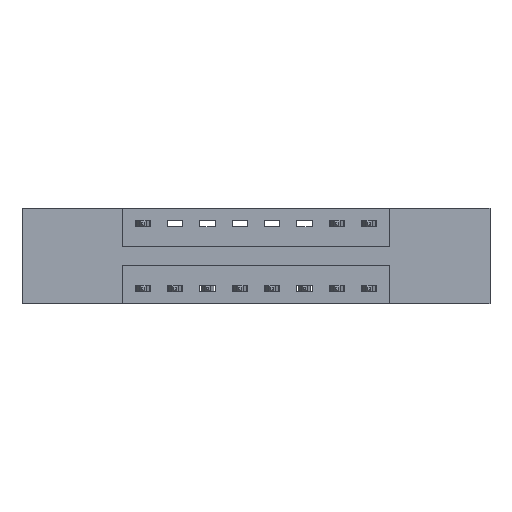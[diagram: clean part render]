
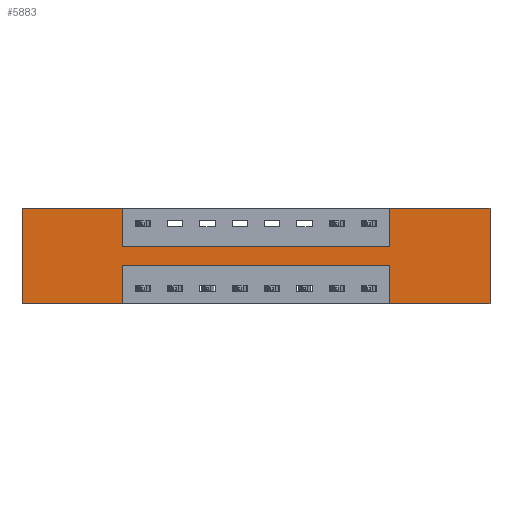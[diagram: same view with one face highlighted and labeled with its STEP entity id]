
A CAD part, front view. The second image highlights one B-rep face of the part: STEP entity #5883.
In plain terms, the highlighted planar face has unit normal (0, -1, 0).
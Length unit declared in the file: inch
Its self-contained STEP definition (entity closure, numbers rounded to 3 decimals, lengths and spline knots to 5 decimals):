
#243 = ORIENTED_EDGE ( 'NONE', *, *, #7865, .F. ) ;
#337 = EDGE_CURVE ( 'NONE', #3674, #3912, #1837, .T. ) ;
#371 = VECTOR ( 'NONE', #8137, 39.37008 ) ;
#409 = VECTOR ( 'NONE', #5251, 39.37008 ) ;
#475 = LINE ( 'NONE', #8628, #8209 ) ;
#596 = VECTOR ( 'NONE', #3770, 39.37008 ) ;
#738 = DIRECTION ( 'NONE',  ( 1., 0., 0. ) ) ;
#795 = CARTESIAN_POINT ( 'NONE',  ( 0.3875, 0., 0. ) ) ;
#803 = CARTESIAN_POINT ( 'NONE',  ( 0., 0., 0. ) ) ;
#1047 = ORIENTED_EDGE ( 'NONE', *, *, #8510, .F. ) ;
#1082 = CARTESIAN_POINT ( 'NONE',  ( 0.3875, 0., -0.37 ) ) ;
#1118 = DIRECTION ( 'NONE',  ( 1., 0., 0. ) ) ;
#1181 = FACE_OUTER_BOUND ( 'NONE', #6843, .T. ) ;
#1190 = ORIENTED_EDGE ( 'NONE', *, *, #1732, .F. ) ;
#1192 = LINE ( 'NONE', #1082, #5356 ) ;
#1216 = ORIENTED_EDGE ( 'NONE', *, *, #2762, .F. ) ;
#1346 = CARTESIAN_POINT ( 'NONE',  ( 0.3875, 0., 0. ) ) ;
#1477 = CARTESIAN_POINT ( 'NONE',  ( 0.3875, 0., -0.22 ) ) ;
#1499 = CARTESIAN_POINT ( 'NONE',  ( 1.4225, 0., 0. ) ) ;
#1594 = VECTOR ( 'NONE', #5205, 39.37008 ) ;
#1732 = EDGE_CURVE ( 'NONE', #6305, #8134, #3743, .T. ) ;
#1837 = LINE ( 'NONE', #803, #9418 ) ;
#1890 = ORIENTED_EDGE ( 'NONE', *, *, #4042, .F. ) ;
#2009 = CARTESIAN_POINT ( 'NONE',  ( 1.4225, 0., -0.22 ) ) ;
#2018 = CARTESIAN_POINT ( 'NONE',  ( 1.4225, 0., -0.37 ) ) ;
#2043 = VERTEX_POINT ( 'NONE', #2009 ) ;
#2159 = ORIENTED_EDGE ( 'NONE', *, *, #337, .F. ) ;
#2162 = VECTOR ( 'NONE', #6125, 39.37008 ) ;
#2228 = ORIENTED_EDGE ( 'NONE', *, *, #9566, .F. ) ;
#2239 = CARTESIAN_POINT ( 'NONE',  ( 0., 0., -0.37 ) ) ;
#2257 = CARTESIAN_POINT ( 'NONE',  ( 1.81, 0., 0. ) ) ;
#2356 = AXIS2_PLACEMENT_3D ( 'NONE', #2239, #7439, #2971 ) ;
#2375 = ORIENTED_EDGE ( 'NONE', *, *, #3370, .F. ) ;
#2468 = VERTEX_POINT ( 'NONE', #9461 ) ;
#2762 = EDGE_CURVE ( 'NONE', #8134, #2468, #7640, .T. ) ;
#2870 = CARTESIAN_POINT ( 'NONE',  ( 0., 0., -0.37 ) ) ;
#2971 = DIRECTION ( 'NONE',  ( 0., 0., -1. ) ) ;
#3019 = CARTESIAN_POINT ( 'NONE',  ( 0.3875, 0., -0.37 ) ) ;
#3094 = ORIENTED_EDGE ( 'NONE', *, *, #4692, .F. ) ;
#3179 = VERTEX_POINT ( 'NONE', #3019 ) ;
#3220 = CARTESIAN_POINT ( 'NONE',  ( 0.3875, 0., -0.15 ) ) ;
#3370 = EDGE_CURVE ( 'NONE', #3179, #3674, #4606, .T. ) ;
#3674 = VERTEX_POINT ( 'NONE', #7063 ) ;
#3743 = LINE ( 'NONE', #795, #9302 ) ;
#3770 = DIRECTION ( 'NONE',  ( -1., 0., 0. ) ) ;
#3912 = VERTEX_POINT ( 'NONE', #6944 ) ;
#4042 = EDGE_CURVE ( 'NONE', #2043, #7553, #5016, .T. ) ;
#4423 = CARTESIAN_POINT ( 'NONE',  ( 1.4225, 0., -0.37 ) ) ;
#4606 = LINE ( 'NONE', #5554, #409 ) ;
#4692 = EDGE_CURVE ( 'NONE', #5772, #8026, #475, .T. ) ;
#4769 = CARTESIAN_POINT ( 'NONE',  ( 1.4225, 0., 0. ) ) ;
#4863 = ORIENTED_EDGE ( 'NONE', *, *, #8646, .F. ) ;
#5016 = LINE ( 'NONE', #1477, #596 ) ;
#5205 = DIRECTION ( 'NONE',  ( 0., 0., 1. ) ) ;
#5251 = DIRECTION ( 'NONE',  ( -1., 0., 0. ) ) ;
#5328 = VECTOR ( 'NONE', #7041, 39.37008 ) ;
#5356 = VECTOR ( 'NONE', #5701, 39.37008 ) ;
#5413 = DIRECTION ( 'NONE',  ( 0., 0., -1. ) ) ;
#5423 = EDGE_CURVE ( 'NONE', #7553, #3179, #1192, .T. ) ;
#5529 = VECTOR ( 'NONE', #6630, 39.37008 ) ;
#5554 = CARTESIAN_POINT ( 'NONE',  ( 0., 0., -0.37 ) ) ;
#5631 = DIRECTION ( 'NONE',  ( 0., 0., 1. ) ) ;
#5651 = VERTEX_POINT ( 'NONE', #8607 ) ;
#5678 = CARTESIAN_POINT ( 'NONE',  ( 0.3875, 0., -0.15 ) ) ;
#5701 = DIRECTION ( 'NONE',  ( 0., 0., -1. ) ) ;
#5772 = VERTEX_POINT ( 'NONE', #4769 ) ;
#5883 = ADVANCED_FACE ( 'NONE', ( #1181 ), #6730, .T. ) ;
#6125 = DIRECTION ( 'NONE',  ( 0., 0., 1. ) ) ;
#6305 = VERTEX_POINT ( 'NONE', #1346 ) ;
#6424 = VECTOR ( 'NONE', #738, 39.37008 ) ;
#6518 = ORIENTED_EDGE ( 'NONE', *, *, #5423, .F. ) ;
#6630 = DIRECTION ( 'NONE',  ( -1., 0., 0. ) ) ;
#6730 = PLANE ( 'NONE',  #2356 ) ;
#6818 = CARTESIAN_POINT ( 'NONE',  ( 0., 0., 0. ) ) ;
#6843 = EDGE_LOOP ( 'NONE', ( #6518, #1890, #2228, #1047, #4863, #3094, #8719, #1216, #1190, #243, #2159, #2375 ) ) ;
#6944 = CARTESIAN_POINT ( 'NONE',  ( 0., 0., 0. ) ) ;
#7024 = EDGE_CURVE ( 'NONE', #2468, #5772, #9672, .T. ) ;
#7041 = DIRECTION ( 'NONE',  ( 1., 0., 0. ) ) ;
#7057 = LINE ( 'NONE', #6818, #6424 ) ;
#7063 = CARTESIAN_POINT ( 'NONE',  ( 0., 0., -0.37 ) ) ;
#7439 = DIRECTION ( 'NONE',  ( 0., -1., 0. ) ) ;
#7553 = VERTEX_POINT ( 'NONE', #9359 ) ;
#7588 = LINE ( 'NONE', #4423, #1594 ) ;
#7640 = LINE ( 'NONE', #3220, #5328 ) ;
#7865 = EDGE_CURVE ( 'NONE', #3912, #6305, #7057, .T. ) ;
#8026 = VERTEX_POINT ( 'NONE', #8347 ) ;
#8134 = VERTEX_POINT ( 'NONE', #5678 ) ;
#8137 = DIRECTION ( 'NONE',  ( 0., 0., -1. ) ) ;
#8209 = VECTOR ( 'NONE', #1118, 39.37008 ) ;
#8347 = CARTESIAN_POINT ( 'NONE',  ( 1.81, 0., 0. ) ) ;
#8386 = VERTEX_POINT ( 'NONE', #2018 ) ;
#8510 = EDGE_CURVE ( 'NONE', #5651, #8386, #9241, .T. ) ;
#8607 = CARTESIAN_POINT ( 'NONE',  ( 1.81, 0., -0.37 ) ) ;
#8628 = CARTESIAN_POINT ( 'NONE',  ( 0., 0., 0. ) ) ;
#8646 = EDGE_CURVE ( 'NONE', #8026, #5651, #8795, .T. ) ;
#8719 = ORIENTED_EDGE ( 'NONE', *, *, #7024, .F. ) ;
#8795 = LINE ( 'NONE', #2257, #371 ) ;
#9241 = LINE ( 'NONE', #2870, #5529 ) ;
#9302 = VECTOR ( 'NONE', #5413, 39.37008 ) ;
#9359 = CARTESIAN_POINT ( 'NONE',  ( 0.3875, 0., -0.22 ) ) ;
#9418 = VECTOR ( 'NONE', #5631, 39.37008 ) ;
#9461 = CARTESIAN_POINT ( 'NONE',  ( 1.4225, 0., -0.15 ) ) ;
#9566 = EDGE_CURVE ( 'NONE', #8386, #2043, #7588, .T. ) ;
#9672 = LINE ( 'NONE', #1499, #2162 ) ;
